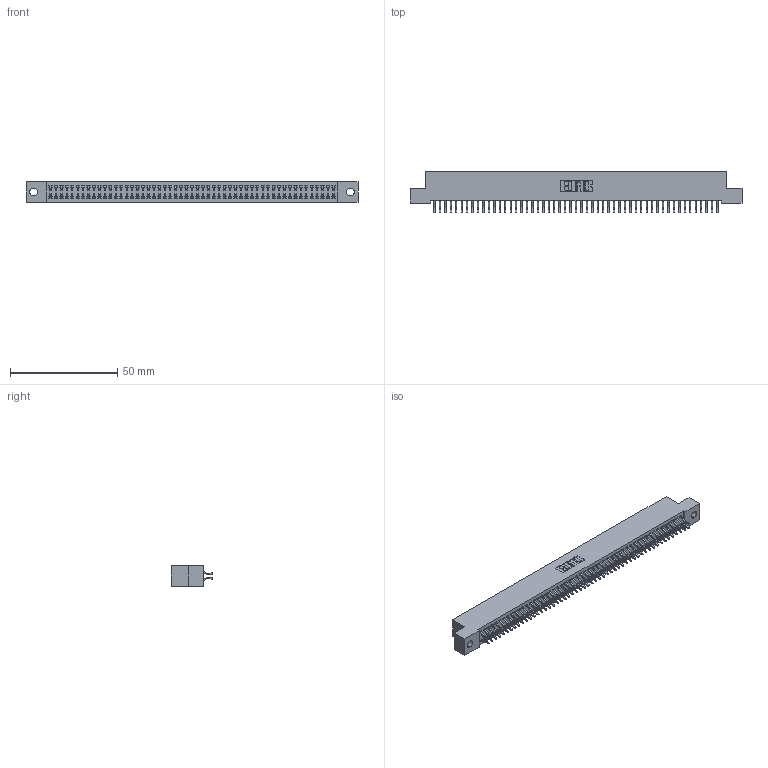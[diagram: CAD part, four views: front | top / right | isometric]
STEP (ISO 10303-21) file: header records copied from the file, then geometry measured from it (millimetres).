
FILE_DESCRIPTION (( 'STEP AP203' ), '1' );
FILE_NAME ('392-106-556-202.STEP', '2019-10-09T22:44:27', ( '' ), ( '' ), 'SwSTEP 2.0', 'SolidWorks 2016', '' );
FILE_SCHEMA (( 'CONFIG_CONTROL_DESIGN' ));
Length unit declared in the file: inch
Products named in the file (3): 342 Part_.128 Slot; 345-292-001_556 Tail; 392-106-556-202
Assembly tree (107 placements, depth 2):
  392-106-556-202
    342 Part_.128 Slot
    345-292-001_556 Tail  x106
Bounding box: 154.94 x 19.58 x 9.4 mm (x, y, z)
Volume: 13918.6 mm3; surface area: 22583.7 mm2
Topology: 107 solids, 107 shells, 6262 faces, 18649 edges, 12290 vertices
Faces by surface type: plane 4310, cylinder 1952
Entity records: 32897 total; most frequent: CARTESIAN_POINT 5454, ORIENTED_EDGE 5378, DIRECTION 4629, EDGE_CURVE 2689, LINE 2553, VECTOR 2553, VERTEX_POINT 1790, AXIS2_PLACEMENT_3D 1038
